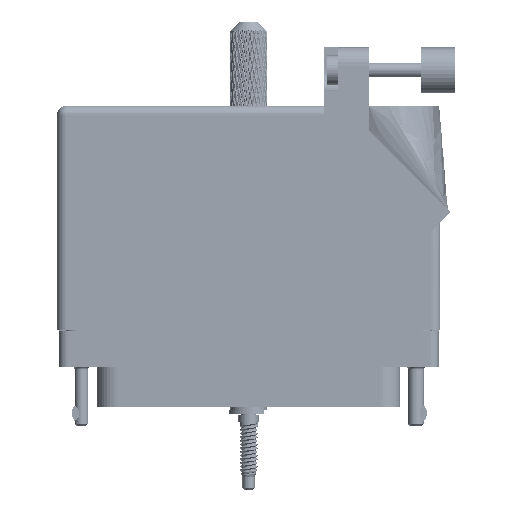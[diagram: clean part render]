
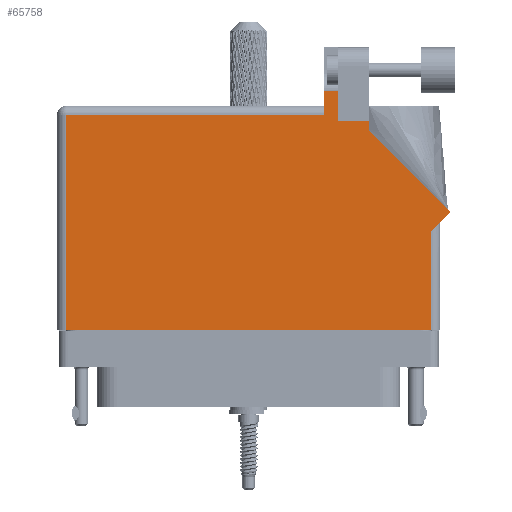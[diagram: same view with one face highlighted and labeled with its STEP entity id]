
A CAD part, front view. The second image highlights one B-rep face of the part: STEP entity #65758.
In plain terms, the highlighted face is planar.
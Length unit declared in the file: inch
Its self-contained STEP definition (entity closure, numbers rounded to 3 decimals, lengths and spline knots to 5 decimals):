
#489 = LINE ( 'NONE', #7092, #95667 ) ;
#677 = DIRECTION ( 'NONE',  ( -1., 0., 0. ) ) ;
#1111 = EDGE_CURVE ( 'NONE', #7743, #94799, #489, .T. ) ;
#1799 = VECTOR ( 'NONE', #27286, 39.37008 ) ;
#3095 = DIRECTION ( 'NONE',  ( -1., 0., 0. ) ) ;
#5777 = CARTESIAN_POINT ( 'NONE',  ( 0.607, 1.33, 0.455 ) ) ;
#6211 = DIRECTION ( 'NONE',  ( 0., 1., 0. ) ) ;
#7092 = CARTESIAN_POINT ( 'NONE',  ( 1.37671, 0.70771, 0.455 ) ) ;
#7743 = VERTEX_POINT ( 'NONE', #34813 ) ;
#8566 = CARTESIAN_POINT ( 'NONE',  ( -1.306, 1.43, 0.455 ) ) ;
#10785 = LINE ( 'NONE', #109995, #50637 ) ;
#11661 = LINE ( 'NONE', #67294, #110101 ) ;
#12240 = DIRECTION ( 'NONE',  ( 0.707, 0.707, 0. ) ) ;
#15560 = CARTESIAN_POINT ( 'NONE',  ( -1.244, -0.1, 0.455 ) ) ;
#16972 = LINE ( 'NONE', #17796, #120094 ) ;
#17796 = CARTESIAN_POINT ( 'NONE',  ( 0.82, 1.33, 0.455 ) ) ;
#20035 = VERTEX_POINT ( 'NONE', #56371 ) ;
#21115 = CARTESIAN_POINT ( 'NONE',  ( -1.306, -0.1, 0.455 ) ) ;
#23525 = VECTOR ( 'NONE', #45900, 39.37008 ) ;
#24093 = CARTESIAN_POINT ( 'NONE',  ( -1.244, -0.1, 0.455 ) ) ;
#25028 = EDGE_LOOP ( 'NONE', ( #43009, #45283, #121253, #50240, #70324, #74240, #68584, #80807, #79746, #104160, #81796 ) ) ;
#25400 = EDGE_CURVE ( 'NONE', #122701, #98253, #121954, .T. ) ;
#25872 = CARTESIAN_POINT ( 'NONE',  ( 0.607, 1.33, 0.455 ) ) ;
#27286 = DIRECTION ( 'NONE',  ( 0., 1., 0. ) ) ;
#29091 = VERTEX_POINT ( 'NONE', #15560 ) ;
#29364 = LINE ( 'NONE', #24093, #66329 ) ;
#29704 = DIRECTION ( 'NONE',  ( 1., 0., 0. ) ) ;
#29898 = AXIS2_PLACEMENT_3D ( 'NONE', #8566, #38044, #106931 ) ;
#34576 = LINE ( 'NONE', #71595, #111716 ) ;
#34813 = CARTESIAN_POINT ( 'NONE',  ( 1.37671, 0.70771, 0.455 ) ) ;
#36696 = LINE ( 'NONE', #45581, #119862 ) ;
#37885 = EDGE_CURVE ( 'NONE', #72601, #29091, #29364, .T. ) ;
#38044 = DIRECTION ( 'NONE',  ( 0., 0., -1. ) ) ;
#43009 = ORIENTED_EDGE ( 'NONE', *, *, #25400, .T. ) ;
#45283 = ORIENTED_EDGE ( 'NONE', *, *, #100772, .T. ) ;
#45581 = CARTESIAN_POINT ( 'NONE',  ( 0.82, 1.26442, 0.455 ) ) ;
#45900 = DIRECTION ( 'NONE',  ( -1., 0., 0. ) ) ;
#46482 = DIRECTION ( 'NONE',  ( 0., -1., 0. ) ) ;
#47875 = FACE_OUTER_BOUND ( 'NONE', #25028, .T. ) ;
#50240 = ORIENTED_EDGE ( 'NONE', *, *, #83923, .T. ) ;
#50637 = VECTOR ( 'NONE', #3095, 39.37008 ) ;
#53127 = CARTESIAN_POINT ( 'NONE',  ( 0.513, 1.5315, 0.455 ) ) ;
#53310 = EDGE_CURVE ( 'NONE', #94799, #116183, #36696, .T. ) ;
#56371 = CARTESIAN_POINT ( 'NONE',  ( 1.244, -0.1, 0.455 ) ) ;
#56380 = DIRECTION ( 'NONE',  ( -0.707, 0.707, 0. ) ) ;
#58645 = EDGE_CURVE ( 'NONE', #29091, #20035, #124501, .T. ) ;
#60815 = CARTESIAN_POINT ( 'NONE',  ( -1.244, 1.368, 0.455 ) ) ;
#63203 = CARTESIAN_POINT ( 'NONE',  ( 0.82, 1.33, 0.455 ) ) ;
#65173 = CARTESIAN_POINT ( 'NONE',  ( 0.82, 1.26442, 0.455 ) ) ;
#65758 = ADVANCED_FACE ( 'NONE', ( #47875 ), #67015, .F. ) ;
#66329 = VECTOR ( 'NONE', #93229, 39.37008 ) ;
#67015 = PLANE ( 'NONE',  #29898 ) ;
#67294 = CARTESIAN_POINT ( 'NONE',  ( 0.513, 1.43, 0.455 ) ) ;
#68584 = ORIENTED_EDGE ( 'NONE', *, *, #112143, .T. ) ;
#70324 = ORIENTED_EDGE ( 'NONE', *, *, #37885, .T. ) ;
#71595 = CARTESIAN_POINT ( 'NONE',  ( 1.306, 0.637, 0.455 ) ) ;
#72601 = VERTEX_POINT ( 'NONE', #60815 ) ;
#74240 = ORIENTED_EDGE ( 'NONE', *, *, #58645, .T. ) ;
#74569 = VERTEX_POINT ( 'NONE', #118330 ) ;
#75014 = DIRECTION ( 'NONE',  ( 0., 1., 0. ) ) ;
#79746 = ORIENTED_EDGE ( 'NONE', *, *, #1111, .T. ) ;
#80091 = EDGE_CURVE ( 'NONE', #74569, #7743, #34576, .T. ) ;
#80807 = ORIENTED_EDGE ( 'NONE', *, *, #80091, .T. ) ;
#81256 = EDGE_CURVE ( 'NONE', #99715, #123284, #11661, .T. ) ;
#81796 = ORIENTED_EDGE ( 'NONE', *, *, #85905, .T. ) ;
#83923 = EDGE_CURVE ( 'NONE', #123284, #72601, #118847, .T. ) ;
#85905 = EDGE_CURVE ( 'NONE', #116183, #122701, #16972, .T. ) ;
#86616 = CARTESIAN_POINT ( 'NONE',  ( 1.244, 0.637, 0.455 ) ) ;
#89358 = LINE ( 'NONE', #86616, #1799 ) ;
#93229 = DIRECTION ( 'NONE',  ( 0., -1., 0. ) ) ;
#94552 = CARTESIAN_POINT ( 'NONE',  ( 0.513, 1.368, 0.455 ) ) ;
#94799 = VERTEX_POINT ( 'NONE', #65173 ) ;
#95667 = VECTOR ( 'NONE', #56380, 39.37008 ) ;
#98253 = VERTEX_POINT ( 'NONE', #126892 ) ;
#99715 = VERTEX_POINT ( 'NONE', #53127 ) ;
#100772 = EDGE_CURVE ( 'NONE', #98253, #99715, #10785, .T. ) ;
#102811 = CARTESIAN_POINT ( 'NONE',  ( -1.306, 1.368, 0.455 ) ) ;
#104160 = ORIENTED_EDGE ( 'NONE', *, *, #53310, .T. ) ;
#104501 = VECTOR ( 'NONE', #29704, 39.37008 ) ;
#106931 = DIRECTION ( 'NONE',  ( -1., 0., 0. ) ) ;
#108134 = VECTOR ( 'NONE', #6211, 39.37008 ) ;
#109995 = CARTESIAN_POINT ( 'NONE',  ( 0.93777, 1.5315, 0.455 ) ) ;
#110101 = VECTOR ( 'NONE', #46482, 39.37008 ) ;
#111716 = VECTOR ( 'NONE', #12240, 39.37008 ) ;
#112143 = EDGE_CURVE ( 'NONE', #20035, #74569, #89358, .T. ) ;
#116183 = VERTEX_POINT ( 'NONE', #63203 ) ;
#118330 = CARTESIAN_POINT ( 'NONE',  ( 1.244, 0.575, 0.455 ) ) ;
#118847 = LINE ( 'NONE', #102811, #23525 ) ;
#119862 = VECTOR ( 'NONE', #75014, 39.37008 ) ;
#120094 = VECTOR ( 'NONE', #677, 39.37008 ) ;
#121253 = ORIENTED_EDGE ( 'NONE', *, *, #81256, .T. ) ;
#121954 = LINE ( 'NONE', #25872, #108134 ) ;
#122701 = VERTEX_POINT ( 'NONE', #5777 ) ;
#123284 = VERTEX_POINT ( 'NONE', #94552 ) ;
#124501 = LINE ( 'NONE', #21115, #104501 ) ;
#126892 = CARTESIAN_POINT ( 'NONE',  ( 0.607, 1.5315, 0.455 ) ) ;
